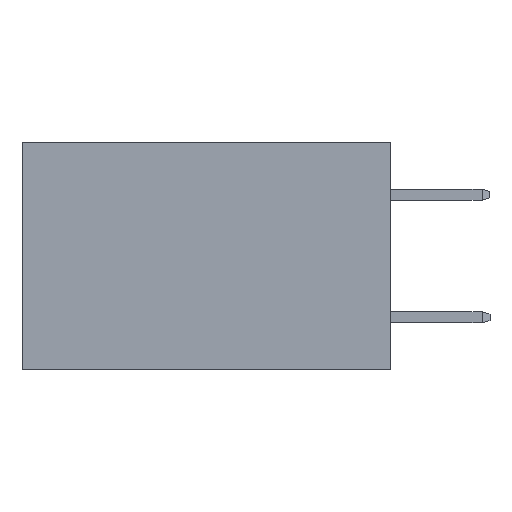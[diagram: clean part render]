
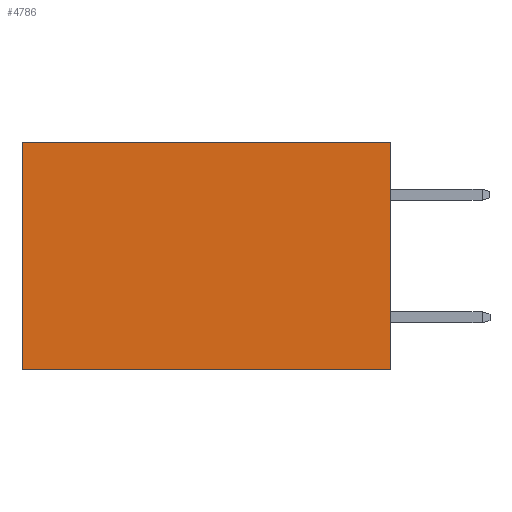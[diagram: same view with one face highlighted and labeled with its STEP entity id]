
A CAD part, left-side view. The second image highlights one B-rep face of the part: STEP entity #4786.
In plain terms, the highlighted planar face has unit normal (-1, 0, 0).
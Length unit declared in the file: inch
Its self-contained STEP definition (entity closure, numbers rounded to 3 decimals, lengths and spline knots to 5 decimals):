
#246 = CARTESIAN_POINT ( 'NONE',  ( 0.2875, 0., 0. ) ) ;
#366 = DIRECTION ( 'NONE',  ( 0., 1., 0. ) ) ;
#630 = DIRECTION ( 'NONE',  ( 1., 0., 0. ) ) ;
#1083 = ORIENTED_EDGE ( 'NONE', *, *, #1175, .T. ) ;
#1175 = EDGE_CURVE ( 'NONE', #7577, #8475, #8697, .T. ) ;
#1978 = CARTESIAN_POINT ( 'NONE',  ( 0.2875, 0.6, 0. ) ) ;
#2116 = EDGE_CURVE ( 'NONE', #8475, #9532, #6757, .T. ) ;
#2342 = VECTOR ( 'NONE', #3487, 39.37008 ) ;
#3400 = ORIENTED_EDGE ( 'NONE', *, *, #2116, .T. ) ;
#3487 = DIRECTION ( 'NONE',  ( 0., 0., -1. ) ) ;
#3534 = AXIS2_PLACEMENT_3D ( 'NONE', #6767, #630, #7785 ) ;
#4112 = CARTESIAN_POINT ( 'NONE',  ( 0.2875, 0.6, -0.37 ) ) ;
#4227 = DIRECTION ( 'NONE',  ( 0., 1., 0. ) ) ;
#4301 = LINE ( 'NONE', #12004, #5590 ) ;
#4361 = ORIENTED_EDGE ( 'NONE', *, *, #6168, .F. ) ;
#4379 = CARTESIAN_POINT ( 'NONE',  ( 0.2875, 0., -0.37 ) ) ;
#4786 = ADVANCED_FACE ( 'NONE', ( #11503 ), #12894, .F. ) ;
#5590 = VECTOR ( 'NONE', #366, 39.37008 ) ;
#6021 = CARTESIAN_POINT ( 'NONE',  ( 0.2875, 0., 0. ) ) ;
#6085 = EDGE_CURVE ( 'NONE', #7577, #9104, #9898, .T. ) ;
#6168 = EDGE_CURVE ( 'NONE', #9104, #9532, #4301, .T. ) ;
#6439 = ORIENTED_EDGE ( 'NONE', *, *, #6085, .F. ) ;
#6757 = LINE ( 'NONE', #1978, #11403 ) ;
#6767 = CARTESIAN_POINT ( 'NONE',  ( 0.2875, 0., 0. ) ) ;
#7390 = CARTESIAN_POINT ( 'NONE',  ( 0.2875, 0., 0. ) ) ;
#7577 = VERTEX_POINT ( 'NONE', #246 ) ;
#7586 = EDGE_LOOP ( 'NONE', ( #3400, #4361, #6439, #1083 ) ) ;
#7785 = DIRECTION ( 'NONE',  ( 0., 0., -1. ) ) ;
#8475 = VERTEX_POINT ( 'NONE', #10555 ) ;
#8697 = LINE ( 'NONE', #6021, #11569 ) ;
#9104 = VERTEX_POINT ( 'NONE', #4379 ) ;
#9221 = DIRECTION ( 'NONE',  ( 0., 0., -1. ) ) ;
#9532 = VERTEX_POINT ( 'NONE', #4112 ) ;
#9898 = LINE ( 'NONE', #7390, #2342 ) ;
#10555 = CARTESIAN_POINT ( 'NONE',  ( 0.2875, 0.6, 0. ) ) ;
#11403 = VECTOR ( 'NONE', #9221, 39.37008 ) ;
#11503 = FACE_OUTER_BOUND ( 'NONE', #7586, .T. ) ;
#11569 = VECTOR ( 'NONE', #4227, 39.37008 ) ;
#12004 = CARTESIAN_POINT ( 'NONE',  ( 0.2875, 0., -0.37 ) ) ;
#12894 = PLANE ( 'NONE',  #3534 ) ;
